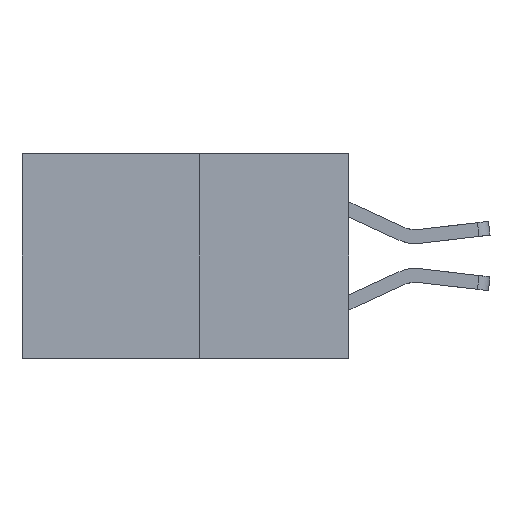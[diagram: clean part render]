
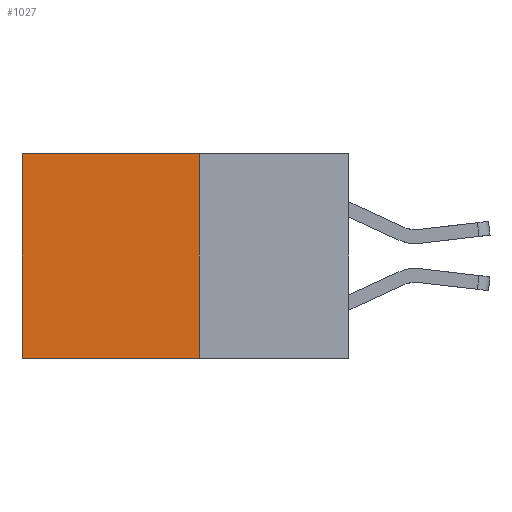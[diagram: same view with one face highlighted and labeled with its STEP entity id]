
A CAD part, left-side view. The second image highlights one B-rep face of the part: STEP entity #1027.
In plain terms, the highlighted planar face has unit normal (-1, 0, 0).
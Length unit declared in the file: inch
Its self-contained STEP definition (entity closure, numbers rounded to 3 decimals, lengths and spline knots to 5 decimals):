
#81 = CARTESIAN_POINT ( 'NONE',  ( 0.277, 0.27, -0.37 ) ) ;
#1023 = VERTEX_POINT ( 'NONE', #9128 ) ;
#1027 = ADVANCED_FACE ( 'NONE', ( #5784 ), #10435, .F. ) ;
#1030 = CARTESIAN_POINT ( 'NONE',  ( 0.277, 0.59, -0.37 ) ) ;
#1565 = EDGE_CURVE ( 'NONE', #3224, #10696, #8005, .T. ) ;
#2831 = VECTOR ( 'NONE', #5043, 39.37008 ) ;
#3163 = VECTOR ( 'NONE', #11775, 39.37008 ) ;
#3224 = VERTEX_POINT ( 'NONE', #12287 ) ;
#3423 = ORIENTED_EDGE ( 'NONE', *, *, #8008, .T. ) ;
#3435 = DIRECTION ( 'NONE',  ( 0., 1., 0. ) ) ;
#3547 = ORIENTED_EDGE ( 'NONE', *, *, #1565, .F. ) ;
#3592 = ORIENTED_EDGE ( 'NONE', *, *, #3684, .F. ) ;
#3628 = ORIENTED_EDGE ( 'NONE', *, *, #4256, .T. ) ;
#3642 = DIRECTION ( 'NONE',  ( 1., 0., 0. ) ) ;
#3684 = EDGE_CURVE ( 'NONE', #11233, #3224, #5564, .T. ) ;
#4256 = EDGE_CURVE ( 'NONE', #11233, #1023, #5902, .T. ) ;
#5043 = DIRECTION ( 'NONE',  ( 0., 0., -1. ) ) ;
#5439 = CARTESIAN_POINT ( 'NONE',  ( 0.277, 0.27, 0. ) ) ;
#5465 = EDGE_LOOP ( 'NONE', ( #3423, #3547, #3592, #3628 ) ) ;
#5489 = VECTOR ( 'NONE', #3435, 39.37008 ) ;
#5564 = LINE ( 'NONE', #6941, #2831 ) ;
#5784 = FACE_OUTER_BOUND ( 'NONE', #5465, .T. ) ;
#5902 = LINE ( 'NONE', #11886, #3163 ) ;
#6474 = LINE ( 'NONE', #1030, #6776 ) ;
#6776 = VECTOR ( 'NONE', #8199, 39.37008 ) ;
#6941 = CARTESIAN_POINT ( 'NONE',  ( 0.277, 0.27, -0.37 ) ) ;
#7912 = CARTESIAN_POINT ( 'NONE',  ( 0.277, 0.59, -0.37 ) ) ;
#8005 = LINE ( 'NONE', #81, #5489 ) ;
#8008 = EDGE_CURVE ( 'NONE', #1023, #10696, #6474, .T. ) ;
#8199 = DIRECTION ( 'NONE',  ( 0., 0., -1. ) ) ;
#9128 = CARTESIAN_POINT ( 'NONE',  ( 0.277, 0.59, 0. ) ) ;
#9168 = AXIS2_PLACEMENT_3D ( 'NONE', #10409, #3642, #9926 ) ;
#9926 = DIRECTION ( 'NONE',  ( 0., 0., -1. ) ) ;
#10409 = CARTESIAN_POINT ( 'NONE',  ( 0.277, 0.27, -0.37 ) ) ;
#10435 = PLANE ( 'NONE',  #9168 ) ;
#10696 = VERTEX_POINT ( 'NONE', #7912 ) ;
#11233 = VERTEX_POINT ( 'NONE', #5439 ) ;
#11775 = DIRECTION ( 'NONE',  ( 0., 1., 0. ) ) ;
#11886 = CARTESIAN_POINT ( 'NONE',  ( 0.277, 0.27, 0. ) ) ;
#12287 = CARTESIAN_POINT ( 'NONE',  ( 0.277, 0.27, -0.37 ) ) ;
